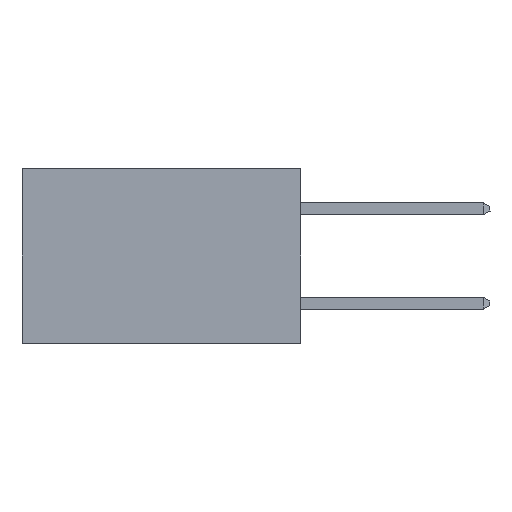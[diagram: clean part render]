
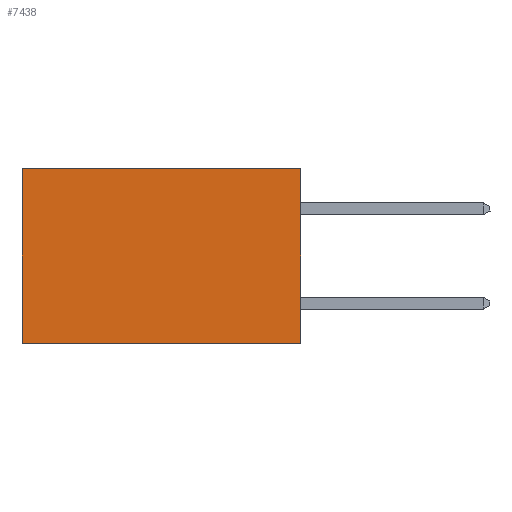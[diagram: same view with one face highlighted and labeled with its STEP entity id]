
A CAD part, left-side view. The second image highlights one B-rep face of the part: STEP entity #7438.
In plain terms, the highlighted planar face has unit normal (-1, 0, 0).
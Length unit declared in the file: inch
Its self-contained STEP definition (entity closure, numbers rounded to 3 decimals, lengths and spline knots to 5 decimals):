
#715 = FACE_OUTER_BOUND ( 'NONE', #14297, .T. ) ;
#795 = EDGE_CURVE ( 'NONE', #8115, #12843, #3505, .T. ) ;
#1270 = VERTEX_POINT ( 'NONE', #2859 ) ;
#1644 = CARTESIAN_POINT ( 'NONE',  ( 0.277, 0., -0.37 ) ) ;
#1963 = VECTOR ( 'NONE', #3625, 39.37008 ) ;
#2502 = CARTESIAN_POINT ( 'NONE',  ( 0.277, 0.59, 0. ) ) ;
#2840 = CARTESIAN_POINT ( 'NONE',  ( 0.277, 0., -0.37 ) ) ;
#2859 = CARTESIAN_POINT ( 'NONE',  ( 0.277, 0.59, -0.37 ) ) ;
#3505 = LINE ( 'NONE', #2840, #10473 ) ;
#3625 = DIRECTION ( 'NONE',  ( 0., 1., 0. ) ) ;
#3746 = CARTESIAN_POINT ( 'NONE',  ( 0.277, 0., 0. ) ) ;
#3901 = EDGE_CURVE ( 'NONE', #12843, #1270, #8893, .T. ) ;
#4129 = ORIENTED_EDGE ( 'NONE', *, *, #15283, .T. ) ;
#4371 = ORIENTED_EDGE ( 'NONE', *, *, #14476, .T. ) ;
#4566 = DIRECTION ( 'NONE',  ( 0., 0., -1. ) ) ;
#5596 = LINE ( 'NONE', #11563, #16174 ) ;
#5744 = VECTOR ( 'NONE', #10467, 39.37008 ) ;
#5808 = ORIENTED_EDGE ( 'NONE', *, *, #795, .F. ) ;
#7438 = ADVANCED_FACE ( 'NONE', ( #715 ), #16095, .F. ) ;
#8115 = VERTEX_POINT ( 'NONE', #8955 ) ;
#8133 = ORIENTED_EDGE ( 'NONE', *, *, #3901, .F. ) ;
#8893 = LINE ( 'NONE', #10695, #5744 ) ;
#8955 = CARTESIAN_POINT ( 'NONE',  ( 0.277, 0., 0. ) ) ;
#10467 = DIRECTION ( 'NONE',  ( 0., 1., 0. ) ) ;
#10473 = VECTOR ( 'NONE', #4566, 39.37008 ) ;
#10695 = CARTESIAN_POINT ( 'NONE',  ( 0.277, 0., -0.37 ) ) ;
#11439 = DIRECTION ( 'NONE',  ( 0., 0., -1. ) ) ;
#11563 = CARTESIAN_POINT ( 'NONE',  ( 0.277, 0.59, -0.37 ) ) ;
#12843 = VERTEX_POINT ( 'NONE', #1644 ) ;
#13433 = AXIS2_PLACEMENT_3D ( 'NONE', #17340, #15914, #16648 ) ;
#13666 = LINE ( 'NONE', #3746, #1963 ) ;
#14297 = EDGE_LOOP ( 'NONE', ( #4129, #8133, #5808, #4371 ) ) ;
#14476 = EDGE_CURVE ( 'NONE', #8115, #14567, #13666, .T. ) ;
#14567 = VERTEX_POINT ( 'NONE', #2502 ) ;
#15283 = EDGE_CURVE ( 'NONE', #14567, #1270, #5596, .T. ) ;
#15914 = DIRECTION ( 'NONE',  ( 1., 0., 0. ) ) ;
#16095 = PLANE ( 'NONE',  #13433 ) ;
#16174 = VECTOR ( 'NONE', #11439, 39.37008 ) ;
#16648 = DIRECTION ( 'NONE',  ( 0., 0., -1. ) ) ;
#17340 = CARTESIAN_POINT ( 'NONE',  ( 0.277, 0., -0.37 ) ) ;
